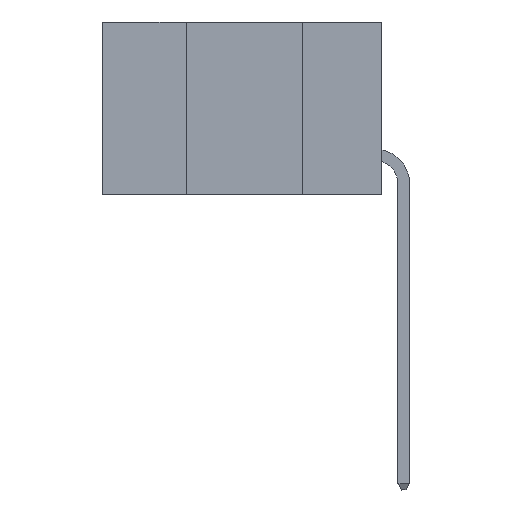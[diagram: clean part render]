
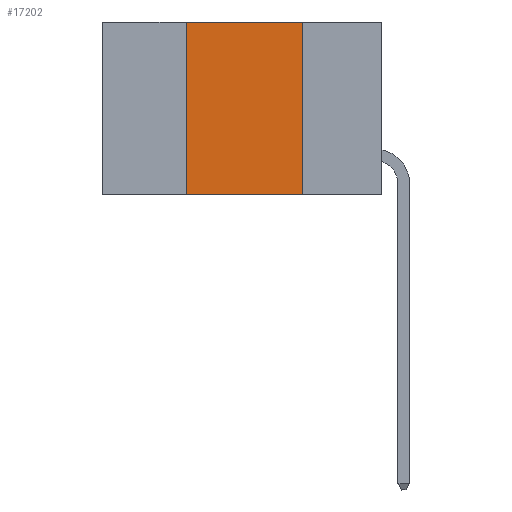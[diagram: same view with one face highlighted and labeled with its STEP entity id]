
A CAD part, left-side view. The second image highlights one B-rep face of the part: STEP entity #17202.
In plain terms, the highlighted planar face has unit normal (-1, 0, 0).
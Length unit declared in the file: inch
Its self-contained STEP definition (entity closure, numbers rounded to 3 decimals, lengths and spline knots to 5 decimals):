
#409 = CARTESIAN_POINT ( 'NONE',  ( 0., 0.17, 0. ) ) ;
#1536 = CARTESIAN_POINT ( 'NONE',  ( 0., 0.42, -0.37 ) ) ;
#2692 = AXIS2_PLACEMENT_3D ( 'NONE', #18381, #22006, #9719 ) ;
#2828 = VECTOR ( 'NONE', #19993, 39.37008 ) ;
#3752 = CARTESIAN_POINT ( 'NONE',  ( 0., 0.17, 0. ) ) ;
#4980 = ORIENTED_EDGE ( 'NONE', *, *, #13875, .F. ) ;
#5488 = EDGE_CURVE ( 'NONE', #9009, #15360, #11427, .T. ) ;
#7276 = CARTESIAN_POINT ( 'NONE',  ( 0., 0.17, -0.37 ) ) ;
#8124 = PLANE ( 'NONE',  #2692 ) ;
#9009 = VERTEX_POINT ( 'NONE', #1536 ) ;
#9269 = VECTOR ( 'NONE', #11222, 39.37008 ) ;
#9719 = DIRECTION ( 'NONE',  ( 0., 0., -1. ) ) ;
#10081 = VECTOR ( 'NONE', #15053, 39.37008 ) ;
#10677 = DIRECTION ( 'NONE',  ( 0., 0., -1. ) ) ;
#11222 = DIRECTION ( 'NONE',  ( 0., -1., 0. ) ) ;
#11427 = LINE ( 'NONE', #16426, #10081 ) ;
#11826 = ORIENTED_EDGE ( 'NONE', *, *, #5488, .T. ) ;
#11827 = LINE ( 'NONE', #3752, #19685 ) ;
#13875 = EDGE_CURVE ( 'NONE', #9009, #21253, #18888, .T. ) ;
#13934 = EDGE_CURVE ( 'NONE', #18333, #15360, #11827, .T. ) ;
#14040 = EDGE_LOOP ( 'NONE', ( #14162, #15945, #4980, #11826 ) ) ;
#14162 = ORIENTED_EDGE ( 'NONE', *, *, #13934, .F. ) ;
#15053 = DIRECTION ( 'NONE',  ( 0., -1., 0. ) ) ;
#15360 = VERTEX_POINT ( 'NONE', #7276 ) ;
#15945 = ORIENTED_EDGE ( 'NONE', *, *, #21630, .F. ) ;
#16426 = CARTESIAN_POINT ( 'NONE',  ( 0., 0.6, -0.37 ) ) ;
#17202 = ADVANCED_FACE ( 'NONE', ( #20560 ), #8124, .F. ) ;
#18203 = CARTESIAN_POINT ( 'NONE',  ( 0., 0.6, 0. ) ) ;
#18272 = CARTESIAN_POINT ( 'NONE',  ( 0., 0.42, 0. ) ) ;
#18333 = VERTEX_POINT ( 'NONE', #409 ) ;
#18381 = CARTESIAN_POINT ( 'NONE',  ( 0., 0.6, 0. ) ) ;
#18888 = LINE ( 'NONE', #18272, #2828 ) ;
#19570 = LINE ( 'NONE', #18203, #9269 ) ;
#19685 = VECTOR ( 'NONE', #10677, 39.37008 ) ;
#19993 = DIRECTION ( 'NONE',  ( 0., 0., 1. ) ) ;
#20560 = FACE_OUTER_BOUND ( 'NONE', #14040, .T. ) ;
#21253 = VERTEX_POINT ( 'NONE', #22211 ) ;
#21630 = EDGE_CURVE ( 'NONE', #21253, #18333, #19570, .T. ) ;
#22006 = DIRECTION ( 'NONE',  ( 1., 0., 0. ) ) ;
#22211 = CARTESIAN_POINT ( 'NONE',  ( 0., 0.42, 0. ) ) ;
